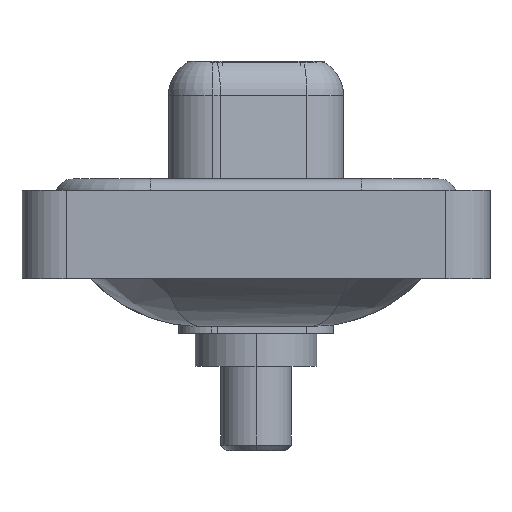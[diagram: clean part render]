
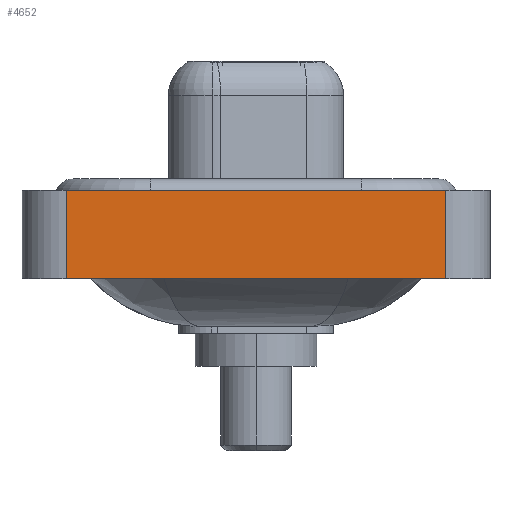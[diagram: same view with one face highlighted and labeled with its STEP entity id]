
A CAD part, left-side view. The second image highlights one B-rep face of the part: STEP entity #4652.
In plain terms, the highlighted planar face has unit normal (-1, 0, 0).
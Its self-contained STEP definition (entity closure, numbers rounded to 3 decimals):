
#808 = EDGE_CURVE ( 'NONE', #3818, #12912, #14419, .T. ) ;
#1208 = CARTESIAN_POINT ( 'NONE',  ( -7.25, 8.55, -3.6 ) ) ;
#1232 = DIRECTION ( 'NONE',  ( 0., 0., 1. ) ) ;
#1239 = DIRECTION ( 'NONE',  ( -1., 0., 0. ) ) ;
#1594 = LINE ( 'NONE', #11050, #12911 ) ;
#1983 = EDGE_CURVE ( 'NONE', #12912, #10848, #13068, .T. ) ;
#2538 = AXIS2_PLACEMENT_3D ( 'NONE', #2748, #1239, #14759 ) ;
#2748 = CARTESIAN_POINT ( 'NONE',  ( -7.25, -8.55, -3.6 ) ) ;
#2827 = PLANE ( 'NONE',  #2538 ) ;
#3588 = CARTESIAN_POINT ( 'NONE',  ( -7.25, -8.55, 0.4 ) ) ;
#3804 = ORIENTED_EDGE ( 'NONE', *, *, #808, .T. ) ;
#3818 = VERTEX_POINT ( 'NONE', #1208 ) ;
#3828 = DIRECTION ( 'NONE',  ( 0., -1., 0. ) ) ;
#4447 = ORIENTED_EDGE ( 'NONE', *, *, #1983, .T. ) ;
#4652 = ADVANCED_FACE ( 'NONE', ( #14844 ), #2827, .T. ) ;
#4929 = CARTESIAN_POINT ( 'NONE',  ( -7.25, -8.55, 0.4 ) ) ;
#5584 = DIRECTION ( 'NONE',  ( 0., 0., 1. ) ) ;
#5893 = DIRECTION ( 'NONE',  ( 0., -1., 0. ) ) ;
#5918 = EDGE_CURVE ( 'NONE', #9716, #10848, #15490, .T. ) ;
#6411 = EDGE_CURVE ( 'NONE', #3818, #9716, #1594, .T. ) ;
#7771 = ORIENTED_EDGE ( 'NONE', *, *, #5918, .F. ) ;
#7832 = CARTESIAN_POINT ( 'NONE',  ( -7.25, -8.55, -3.6 ) ) ;
#8232 = CARTESIAN_POINT ( 'NONE',  ( -7.25, -8.55, -3.6 ) ) ;
#8922 = VECTOR ( 'NONE', #5584, 1000. ) ;
#9716 = VERTEX_POINT ( 'NONE', #11660 ) ;
#10848 = VERTEX_POINT ( 'NONE', #4929 ) ;
#11050 = CARTESIAN_POINT ( 'NONE',  ( -7.25, 8.55, -3.6 ) ) ;
#11660 = CARTESIAN_POINT ( 'NONE',  ( -7.25, 8.55, 0.4 ) ) ;
#11671 = CARTESIAN_POINT ( 'NONE',  ( -7.25, -8.55, -3.6 ) ) ;
#12911 = VECTOR ( 'NONE', #1232, 1000. ) ;
#12912 = VERTEX_POINT ( 'NONE', #11671 ) ;
#13068 = LINE ( 'NONE', #7832, #8922 ) ;
#14280 = VECTOR ( 'NONE', #5893, 1000. ) ;
#14419 = LINE ( 'NONE', #8232, #14280 ) ;
#14431 = VECTOR ( 'NONE', #3828, 1000. ) ;
#14759 = DIRECTION ( 'NONE',  ( 0., 0., 1. ) ) ;
#14844 = FACE_OUTER_BOUND ( 'NONE', #15301, .T. ) ;
#15209 = ORIENTED_EDGE ( 'NONE', *, *, #6411, .F. ) ;
#15301 = EDGE_LOOP ( 'NONE', ( #4447, #7771, #15209, #3804 ) ) ;
#15490 = LINE ( 'NONE', #3588, #14431 ) ;
